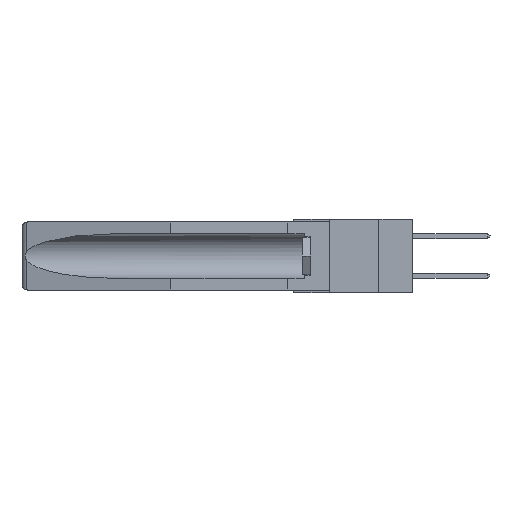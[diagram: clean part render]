
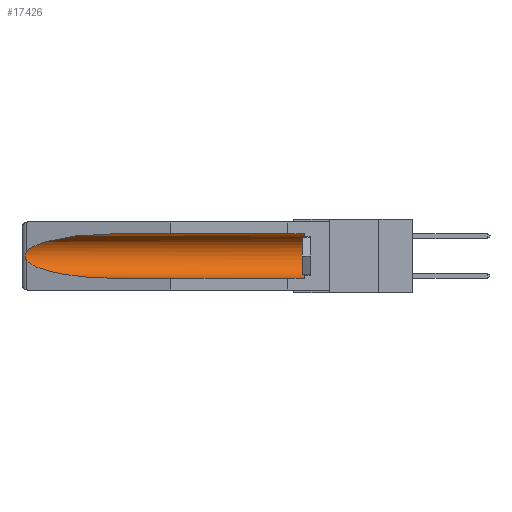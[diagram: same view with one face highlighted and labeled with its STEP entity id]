
A CAD part, left-side view. The second image highlights one B-rep face of the part: STEP entity #17426.
In plain terms, the highlighted cylindrical face has radius 2.857 mm (diameter 5.715 mm), a partial arc.
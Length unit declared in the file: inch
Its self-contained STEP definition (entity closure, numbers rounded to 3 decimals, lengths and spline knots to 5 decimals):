
#392 = CYLINDRICAL_SURFACE ( 'NONE', #15142, 0.1125 ) ;
#668 = ORIENTED_EDGE ( 'NONE', *, *, #14943, .T. ) ;
#955 =( BOUNDED_CURVE ( )  B_SPLINE_CURVE ( 3, ( #2622, #19884, #22173, #2730 ),
 .UNSPECIFIED., .F., .T. ) 
 B_SPLINE_CURVE_WITH_KNOTS ( ( 4, 4 ),
 ( 0.1948, 1.5708 ),
 .UNSPECIFIED. ) 
 CURVE ( )  GEOMETRIC_REPRESENTATION_ITEM ( )  RATIONAL_B_SPLINE_CURVE ( ( 1., 0.848, 0.848, 1. ) ) 
 REPRESENTATION_ITEM ( '' )  );
#1082 = CARTESIAN_POINT ( 'NONE',  ( 0.26654, 1.53092, -0.15636 ) ) ;
#1204 = CARTESIAN_POINT ( 'NONE',  ( 0.2675, 1.53308, -0.17534 ) ) ;
#2264 = VERTEX_POINT ( 'NONE', #18653 ) ;
#2622 = CARTESIAN_POINT ( 'NONE',  ( 0.26537, 1.52718, -0.19328 ) ) ;
#2624 = DIRECTION ( 'NONE',  ( 0., 0., 1. ) ) ;
#2653 = VERTEX_POINT ( 'NONE', #29346 ) ;
#2730 = CARTESIAN_POINT ( 'NONE',  ( 0.155, 1.07973, -0.284 ) ) ;
#2853 = CARTESIAN_POINT ( 'NONE',  ( 0.155, 1.07973, -0.284 ) ) ;
#3290 = CARTESIAN_POINT ( 'NONE',  ( 0.155, 1.07973, -0.059 ) ) ;
#3504 = CARTESIAN_POINT ( 'NONE',  ( 0.21114, 1.30732, -0.059 ) ) ;
#3747 = VERTEX_POINT ( 'NONE', #2853 ) ;
#6509 = VERTEX_POINT ( 'NONE', #10395 ) ;
#6746 = DIRECTION ( 'NONE',  ( 0., 0., 1. ) ) ;
#7603 = CIRCLE ( 'NONE', #26405, 0.1125 ) ;
#7675 = CARTESIAN_POINT ( 'NONE',  ( 0.155, -0.30754, -0.059 ) ) ;
#9369 = LINE ( 'NONE', #7675, #20124 ) ;
#9441 = CARTESIAN_POINT ( 'NONE',  ( 0.26597, 1.5296, -0.19026 ) ) ;
#10395 = CARTESIAN_POINT ( 'NONE',  ( 0.26537, 1.52718, -0.14972 ) ) ;
#11530 =( BOUNDED_CURVE ( )  B_SPLINE_CURVE ( 3, ( #28511, #3504, #13758, #16255 ),
 .UNSPECIFIED., .F., .F. ) 
 B_SPLINE_CURVE_WITH_KNOTS ( ( 4, 4 ),
 ( 4.71239, 6.08839 ),
 .UNSPECIFIED. ) 
 CURVE ( )  GEOMETRIC_REPRESENTATION_ITEM ( )  RATIONAL_B_SPLINE_CURVE ( ( 1., 0.848, 0.848, 1. ) ) 
 REPRESENTATION_ITEM ( '' )  );
#12172 = CARTESIAN_POINT ( 'NONE',  ( 0.26537, 1.52718, -0.19328 ) ) ;
#12241 = DIRECTION ( 'NONE',  ( 0., 1., 0. ) ) ;
#12370 = EDGE_CURVE ( 'NONE', #2653, #3747, #23457, .T. ) ;
#12735 = DIRECTION ( 'NONE',  ( 0., 1., 0. ) ) ;
#13645 = EDGE_CURVE ( 'NONE', #2653, #2264, #7603, .T. ) ;
#13758 = CARTESIAN_POINT ( 'NONE',  ( 0.25451, 1.48313, -0.09465 ) ) ;
#14305 = CARTESIAN_POINT ( 'NONE',  ( 0.26655, 1.53094, -0.18657 ) ) ;
#14943 = EDGE_CURVE ( 'NONE', #30935, #6509, #11530, .T. ) ;
#15142 = AXIS2_PLACEMENT_3D ( 'NONE', #26658, #29655, #6746 ) ;
#15431 = B_SPLINE_CURVE_WITH_KNOTS ( 'NONE', 3,
 ( #18711, #30631, #1082, #15905, #18385, #1204, #19130, #14305, #9441, #16984 ),
 .UNSPECIFIED., .F., .F.,
 ( 4, 2, 2, 2, 4 ),
 ( 0., 0.00029, 0.00058, 0.00087, 0.00117 ),
 .UNSPECIFIED. ) ;
#15905 = CARTESIAN_POINT ( 'NONE',  ( 0.2673, 1.5327, -0.16383 ) ) ;
#16255 = CARTESIAN_POINT ( 'NONE',  ( 0.26537, 1.52718, -0.14972 ) ) ;
#16667 = EDGE_LOOP ( 'NONE', ( #668, #25568, #27698, #26306, #17915, #26795 ) ) ;
#16984 = CARTESIAN_POINT ( 'NONE',  ( 0.26537, 1.52718, -0.19328 ) ) ;
#17426 = ADVANCED_FACE ( 'NONE', ( #23255 ), #392, .F. ) ;
#17915 = ORIENTED_EDGE ( 'NONE', *, *, #13645, .T. ) ;
#18385 = CARTESIAN_POINT ( 'NONE',  ( 0.2675, 1.53308, -0.16763 ) ) ;
#18653 = CARTESIAN_POINT ( 'NONE',  ( 0.155, 0.126, -0.059 ) ) ;
#18711 = CARTESIAN_POINT ( 'NONE',  ( 0.26537, 1.52718, -0.14972 ) ) ;
#19130 = CARTESIAN_POINT ( 'NONE',  ( 0.2673, 1.53269, -0.17917 ) ) ;
#19251 = VERTEX_POINT ( 'NONE', #12172 ) ;
#19554 = DIRECTION ( 'NONE',  ( 0., -1., 0. ) ) ;
#19884 = CARTESIAN_POINT ( 'NONE',  ( 0.25451, 1.48313, -0.24835 ) ) ;
#20124 = VECTOR ( 'NONE', #12735, 39.37008 ) ;
#20788 = EDGE_CURVE ( 'NONE', #19251, #3747, #955, .T. ) ;
#22173 = CARTESIAN_POINT ( 'NONE',  ( 0.21114, 1.30732, -0.284 ) ) ;
#23255 = FACE_OUTER_BOUND ( 'NONE', #16667, .T. ) ;
#23457 = LINE ( 'NONE', #24818, #29178 ) ;
#24818 = CARTESIAN_POINT ( 'NONE',  ( 0.155, -0.30754, -0.284 ) ) ;
#24841 = CARTESIAN_POINT ( 'NONE',  ( 0.155, 0.126, -0.1715 ) ) ;
#25568 = ORIENTED_EDGE ( 'NONE', *, *, #28462, .T. ) ;
#26306 = ORIENTED_EDGE ( 'NONE', *, *, #12370, .F. ) ;
#26405 = AXIS2_PLACEMENT_3D ( 'NONE', #24841, #19554, #2624 ) ;
#26658 = CARTESIAN_POINT ( 'NONE',  ( 0.155, -0.30754, -0.1715 ) ) ;
#26795 = ORIENTED_EDGE ( 'NONE', *, *, #31373, .T. ) ;
#27698 = ORIENTED_EDGE ( 'NONE', *, *, #20788, .T. ) ;
#28462 = EDGE_CURVE ( 'NONE', #6509, #19251, #15431, .T. ) ;
#28511 = CARTESIAN_POINT ( 'NONE',  ( 0.155, 1.07973, -0.059 ) ) ;
#29178 = VECTOR ( 'NONE', #12241, 39.37008 ) ;
#29346 = CARTESIAN_POINT ( 'NONE',  ( 0.155, 0.126, -0.284 ) ) ;
#29655 = DIRECTION ( 'NONE',  ( 0., 1., 0. ) ) ;
#30631 = CARTESIAN_POINT ( 'NONE',  ( 0.26597, 1.52961, -0.15275 ) ) ;
#30935 = VERTEX_POINT ( 'NONE', #3290 ) ;
#31373 = EDGE_CURVE ( 'NONE', #2264, #30935, #9369, .T. ) ;
